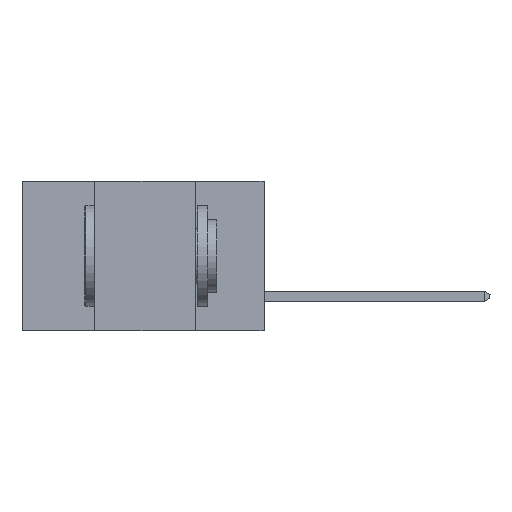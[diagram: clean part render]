
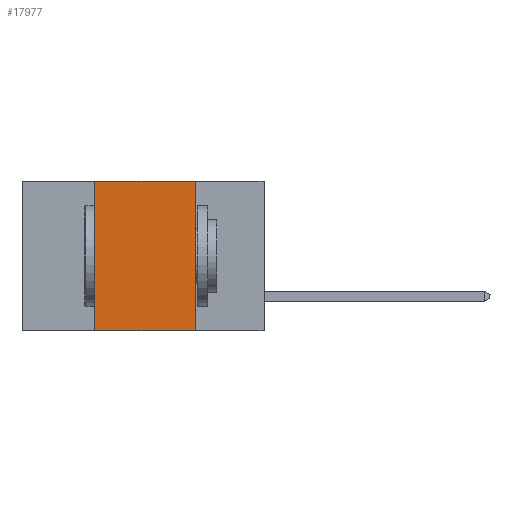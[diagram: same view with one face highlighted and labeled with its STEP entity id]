
A CAD part, left-side view. The second image highlights one B-rep face of the part: STEP entity #17977.
In plain terms, the highlighted planar face has unit normal (-1, 0, 0).
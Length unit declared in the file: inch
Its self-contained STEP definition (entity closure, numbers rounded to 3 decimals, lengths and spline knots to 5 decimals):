
#1164 = CARTESIAN_POINT ( 'NONE',  ( 0., 0.6, 0. ) ) ;
#2388 = CARTESIAN_POINT ( 'NONE',  ( 0., 0.42, -0.37 ) ) ;
#2750 = ORIENTED_EDGE ( 'NONE', *, *, #16103, .F. ) ;
#2881 = VECTOR ( 'NONE', #8407, 39.37008 ) ;
#3817 = CARTESIAN_POINT ( 'NONE',  ( 0., 0.42, 0. ) ) ;
#5122 = VERTEX_POINT ( 'NONE', #24397 ) ;
#5444 = LINE ( 'NONE', #1164, #17155 ) ;
#5683 = CARTESIAN_POINT ( 'NONE',  ( 0., 0.17, -0.37 ) ) ;
#5739 = CARTESIAN_POINT ( 'NONE',  ( 0., 0.17, 0. ) ) ;
#5740 = EDGE_CURVE ( 'NONE', #5122, #16630, #12407, .T. ) ;
#5887 = ORIENTED_EDGE ( 'NONE', *, *, #24059, .F. ) ;
#8394 = DIRECTION ( 'NONE',  ( 0., -1., 0. ) ) ;
#8407 = DIRECTION ( 'NONE',  ( 0., 0., 1. ) ) ;
#9061 = VERTEX_POINT ( 'NONE', #5739 ) ;
#11273 = CARTESIAN_POINT ( 'NONE',  ( 0., 0.17, -0.37 ) ) ;
#11434 = PLANE ( 'NONE',  #26010 ) ;
#11575 = DIRECTION ( 'NONE',  ( 0., 0., -1. ) ) ;
#11716 = LINE ( 'NONE', #5683, #14533 ) ;
#12407 = LINE ( 'NONE', #20624, #17751 ) ;
#13019 = ORIENTED_EDGE ( 'NONE', *, *, #5740, .T. ) ;
#13622 = DIRECTION ( 'NONE',  ( 0., -1., 0. ) ) ;
#14533 = VECTOR ( 'NONE', #19780, 39.37008 ) ;
#14792 = ORIENTED_EDGE ( 'NONE', *, *, #21062, .F. ) ;
#16103 = EDGE_CURVE ( 'NONE', #5122, #19337, #16467, .T. ) ;
#16467 = LINE ( 'NONE', #2388, #2881 ) ;
#16630 = VERTEX_POINT ( 'NONE', #11273 ) ;
#17155 = VECTOR ( 'NONE', #13622, 39.37008 ) ;
#17751 = VECTOR ( 'NONE', #8394, 39.37008 ) ;
#17977 = ADVANCED_FACE ( 'NONE', ( #22201 ), #11434, .F. ) ;
#19337 = VERTEX_POINT ( 'NONE', #3817 ) ;
#19652 = DIRECTION ( 'NONE',  ( 1., 0., 0. ) ) ;
#19780 = DIRECTION ( 'NONE',  ( 0., 0., -1. ) ) ;
#19860 = EDGE_LOOP ( 'NONE', ( #14792, #5887, #2750, #13019 ) ) ;
#20624 = CARTESIAN_POINT ( 'NONE',  ( 0., 0.6, -0.37 ) ) ;
#21062 = EDGE_CURVE ( 'NONE', #9061, #16630, #11716, .T. ) ;
#21797 = CARTESIAN_POINT ( 'NONE',  ( 0., 0.6, 0. ) ) ;
#22201 = FACE_OUTER_BOUND ( 'NONE', #19860, .T. ) ;
#24059 = EDGE_CURVE ( 'NONE', #19337, #9061, #5444, .T. ) ;
#24397 = CARTESIAN_POINT ( 'NONE',  ( 0., 0.42, -0.37 ) ) ;
#26010 = AXIS2_PLACEMENT_3D ( 'NONE', #21797, #19652, #11575 ) ;
